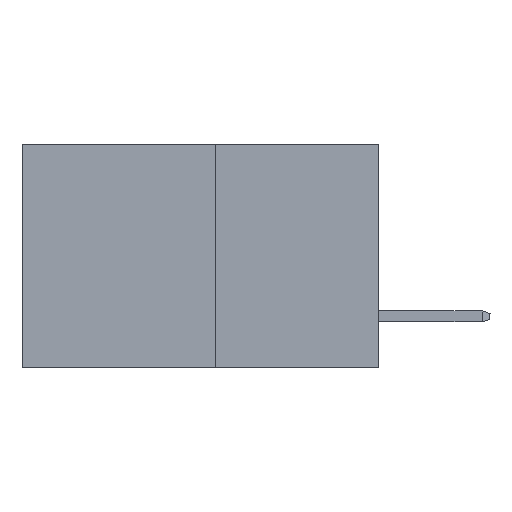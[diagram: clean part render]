
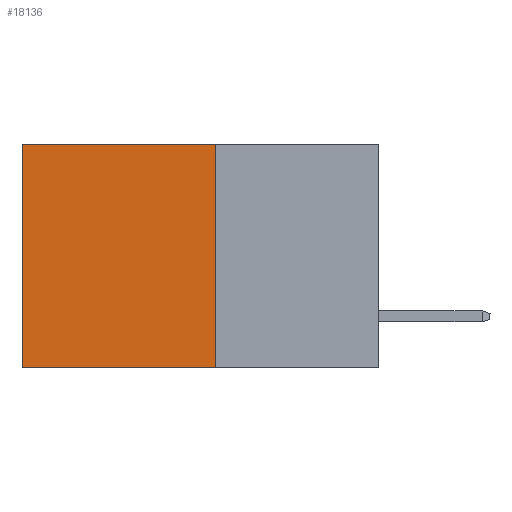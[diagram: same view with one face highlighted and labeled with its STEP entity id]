
A CAD part, left-side view. The second image highlights one B-rep face of the part: STEP entity #18136.
In plain terms, the highlighted planar face has unit normal (-1, 0, 0).
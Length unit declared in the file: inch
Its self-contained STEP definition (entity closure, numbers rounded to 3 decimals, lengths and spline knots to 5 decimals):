
#248 = VERTEX_POINT ( 'NONE', #4943 ) ;
#1555 = CARTESIAN_POINT ( 'NONE',  ( 0.277, 0.27, 0. ) ) ;
#4590 = VERTEX_POINT ( 'NONE', #9943 ) ;
#4684 = VERTEX_POINT ( 'NONE', #24177 ) ;
#4943 = CARTESIAN_POINT ( 'NONE',  ( 0.277, 0.59, 0. ) ) ;
#5651 = LINE ( 'NONE', #14363, #29334 ) ;
#5926 = DIRECTION ( 'NONE',  ( 0., 0., -1. ) ) ;
#5994 = PLANE ( 'NONE',  #22915 ) ;
#6022 = CARTESIAN_POINT ( 'NONE',  ( 0.277, 0.27, -0.37 ) ) ;
#6292 = DIRECTION ( 'NONE',  ( 1., 0., 0. ) ) ;
#9066 = EDGE_LOOP ( 'NONE', ( #9588, #21137, #22618, #28463 ) ) ;
#9588 = ORIENTED_EDGE ( 'NONE', *, *, #11559, .T. ) ;
#9889 = VERTEX_POINT ( 'NONE', #18699 ) ;
#9943 = CARTESIAN_POINT ( 'NONE',  ( 0.277, 0.27, -0.37 ) ) ;
#10142 = LINE ( 'NONE', #1555, #28245 ) ;
#11559 = EDGE_CURVE ( 'NONE', #248, #4684, #18604, .T. ) ;
#12940 = DIRECTION ( 'NONE',  ( 0., 0., -1. ) ) ;
#14363 = CARTESIAN_POINT ( 'NONE',  ( 0.277, 0.27, -0.37 ) ) ;
#16764 = DIRECTION ( 'NONE',  ( 0., 1., 0. ) ) ;
#17661 = VECTOR ( 'NONE', #12940, 39.37008 ) ;
#18136 = ADVANCED_FACE ( 'NONE', ( #30518 ), #5994, .F. ) ;
#18604 = LINE ( 'NONE', #27100, #24069 ) ;
#18699 = CARTESIAN_POINT ( 'NONE',  ( 0.277, 0.27, 0. ) ) ;
#21137 = ORIENTED_EDGE ( 'NONE', *, *, #26658, .F. ) ;
#21386 = EDGE_CURVE ( 'NONE', #9889, #4590, #28626, .T. ) ;
#22034 = EDGE_CURVE ( 'NONE', #9889, #248, #10142, .T. ) ;
#22618 = ORIENTED_EDGE ( 'NONE', *, *, #21386, .F. ) ;
#22915 = AXIS2_PLACEMENT_3D ( 'NONE', #6022, #6292, #5926 ) ;
#23158 = DIRECTION ( 'NONE',  ( 0., 1., 0. ) ) ;
#24069 = VECTOR ( 'NONE', #29028, 39.37008 ) ;
#24177 = CARTESIAN_POINT ( 'NONE',  ( 0.277, 0.59, -0.37 ) ) ;
#24672 = CARTESIAN_POINT ( 'NONE',  ( 0.277, 0.27, -0.37 ) ) ;
#26658 = EDGE_CURVE ( 'NONE', #4590, #4684, #5651, .T. ) ;
#27100 = CARTESIAN_POINT ( 'NONE',  ( 0.277, 0.59, -0.37 ) ) ;
#28245 = VECTOR ( 'NONE', #23158, 39.37008 ) ;
#28463 = ORIENTED_EDGE ( 'NONE', *, *, #22034, .T. ) ;
#28626 = LINE ( 'NONE', #24672, #17661 ) ;
#29028 = DIRECTION ( 'NONE',  ( 0., 0., -1. ) ) ;
#29334 = VECTOR ( 'NONE', #16764, 39.37008 ) ;
#30518 = FACE_OUTER_BOUND ( 'NONE', #9066, .T. ) ;
